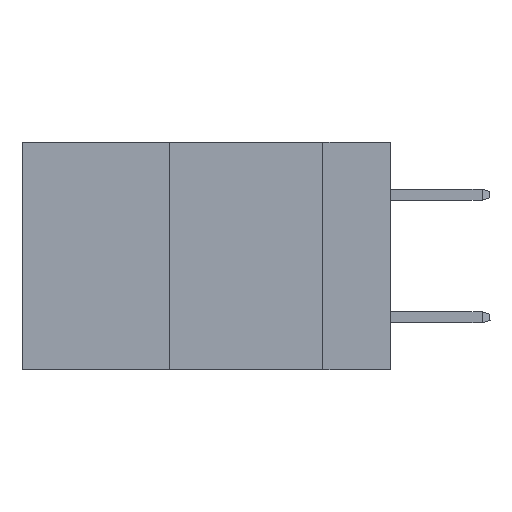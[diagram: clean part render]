
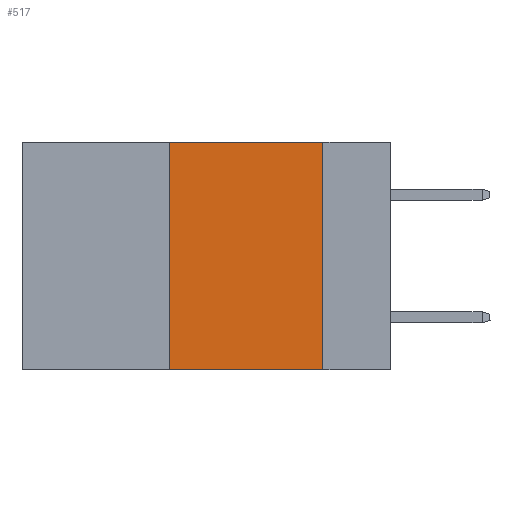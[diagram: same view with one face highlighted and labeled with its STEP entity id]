
A CAD part, left-side view. The second image highlights one B-rep face of the part: STEP entity #517.
In plain terms, the highlighted planar face has unit normal (-1, 0, 0).
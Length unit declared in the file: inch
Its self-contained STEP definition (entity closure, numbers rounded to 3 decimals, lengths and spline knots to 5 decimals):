
#517 = ADVANCED_FACE ( 'NONE', ( #622 ), #4093, .F. ) ;
#622 = FACE_OUTER_BOUND ( 'NONE', #7403, .T. ) ;
#833 = ORIENTED_EDGE ( 'NONE', *, *, #6911, .T. ) ;
#846 = EDGE_CURVE ( 'NONE', #3334, #3646, #7124, .T. ) ;
#1553 = CARTESIAN_POINT ( 'NONE',  ( 0., 0.36, 0. ) ) ;
#2156 = DIRECTION ( 'NONE',  ( 0., -1., 0. ) ) ;
#2534 = VECTOR ( 'NONE', #8690, 39.37008 ) ;
#2613 = CARTESIAN_POINT ( 'NONE',  ( 0., 0.36, 0. ) ) ;
#2969 = VECTOR ( 'NONE', #5856, 39.37008 ) ;
#3284 = LINE ( 'NONE', #9864, #5373 ) ;
#3334 = VERTEX_POINT ( 'NONE', #8793 ) ;
#3646 = VERTEX_POINT ( 'NONE', #5973 ) ;
#4093 = PLANE ( 'NONE',  #8010 ) ;
#4430 = ORIENTED_EDGE ( 'NONE', *, *, #8893, .F. ) ;
#4438 = CARTESIAN_POINT ( 'NONE',  ( 0., 0.11, 0. ) ) ;
#4703 = LINE ( 'NONE', #1553, #2534 ) ;
#4725 = DIRECTION ( 'NONE',  ( 1., 0., 0. ) ) ;
#4900 = ORIENTED_EDGE ( 'NONE', *, *, #8488, .F. ) ;
#5226 = DIRECTION ( 'NONE',  ( 0., -1., 0. ) ) ;
#5373 = VECTOR ( 'NONE', #5226, 39.37008 ) ;
#5445 = VERTEX_POINT ( 'NONE', #6474 ) ;
#5820 = DIRECTION ( 'NONE',  ( 0., 0., -1. ) ) ;
#5856 = DIRECTION ( 'NONE',  ( 0., 0., -1. ) ) ;
#5973 = CARTESIAN_POINT ( 'NONE',  ( 0., 0.11, -0.37 ) ) ;
#6474 = CARTESIAN_POINT ( 'NONE',  ( 0., 0.36, -0.37 ) ) ;
#6587 = CARTESIAN_POINT ( 'NONE',  ( 0., 0.6, 0. ) ) ;
#6614 = VECTOR ( 'NONE', #2156, 39.37008 ) ;
#6911 = EDGE_CURVE ( 'NONE', #5445, #3646, #8971, .T. ) ;
#7124 = LINE ( 'NONE', #4438, #2969 ) ;
#7290 = VERTEX_POINT ( 'NONE', #2613 ) ;
#7403 = EDGE_LOOP ( 'NONE', ( #10074, #4430, #4900, #833 ) ) ;
#8010 = AXIS2_PLACEMENT_3D ( 'NONE', #6587, #4725, #5820 ) ;
#8488 = EDGE_CURVE ( 'NONE', #5445, #7290, #4703, .T. ) ;
#8690 = DIRECTION ( 'NONE',  ( 0., 0., 1. ) ) ;
#8793 = CARTESIAN_POINT ( 'NONE',  ( 0., 0.11, 0. ) ) ;
#8893 = EDGE_CURVE ( 'NONE', #7290, #3334, #3284, .T. ) ;
#8971 = LINE ( 'NONE', #9207, #6614 ) ;
#9207 = CARTESIAN_POINT ( 'NONE',  ( 0., 0.6, -0.37 ) ) ;
#9864 = CARTESIAN_POINT ( 'NONE',  ( 0., 0.6, 0. ) ) ;
#10074 = ORIENTED_EDGE ( 'NONE', *, *, #846, .F. ) ;
